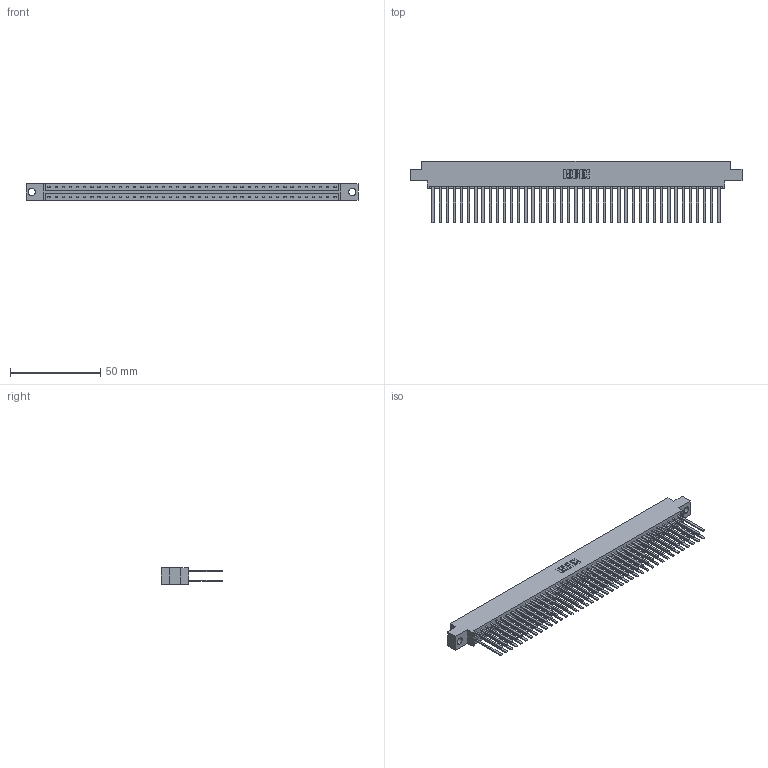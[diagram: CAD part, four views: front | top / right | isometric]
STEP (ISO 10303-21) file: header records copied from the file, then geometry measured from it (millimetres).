
FILE_DESCRIPTION (( 'STEP AP203' ), '1' );
FILE_NAME ('833-082-544-804.STEP', '2020-06-05T23:59:30', ( '' ), ( '' ), 'SwSTEP 2.0', 'SolidWorks 2020', '' );
FILE_SCHEMA (( 'CONFIG_CONTROL_DESIGN' ));
Length unit declared in the file: inch
Products named in the file (3): 833-082-544-804; 345-292-001_345-293-144; 833 Part_Offset - .156 Dia - TH
Assembly tree (83 placements, depth 2):
  833-082-544-804
    833 Part_Offset - .156 Dia - TH
    345-292-001_345-293-144  x82
Bounding box: 184 x 34.3 x 9.4 mm (x, y, z)
Volume: 19609.6 mm3; surface area: 26894 mm2
Topology: 83 solids, 83 shells, 3890 faces, 11557 edges, 7594 vertices
Faces by surface type: plane 2698, cylinder 1192
Entity records: 26457 total; most frequent: CARTESIAN_POINT 4386, ORIENTED_EDGE 4322, DIRECTION 3745, EDGE_CURVE 2161, VECTOR 2037, LINE 2037, VERTEX_POINT 1438, AXIS2_PLACEMENT_3D 854
